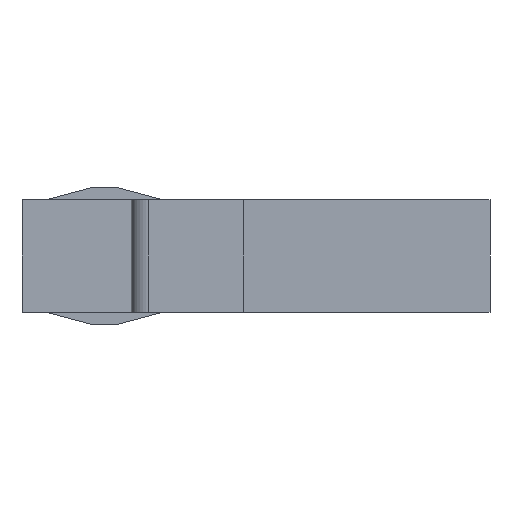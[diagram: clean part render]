
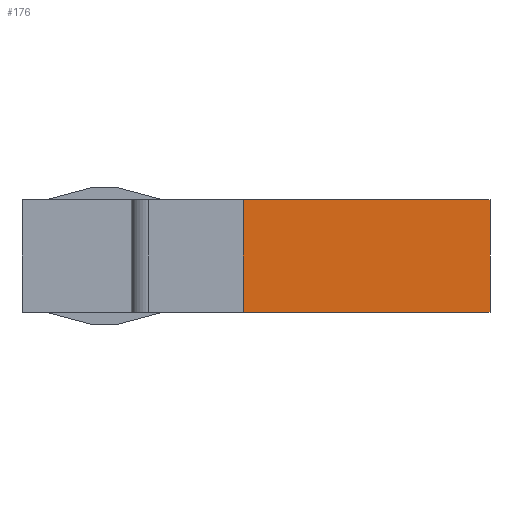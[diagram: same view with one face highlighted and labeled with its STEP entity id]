
A CAD part, left-side view. The second image highlights one B-rep face of the part: STEP entity #176.
In plain terms, the highlighted planar face has unit normal (-1, 0, 0).
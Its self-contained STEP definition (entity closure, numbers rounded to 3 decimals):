
#112 = FACE_OUTER_BOUND ( 'NONE', #405, .T. ) ;
#115 = ORIENTED_EDGE ( 'NONE', *, *, #142, .T. ) ;
#142 = EDGE_CURVE ( 'NONE', #905, #1767, #2941, .T. ) ;
#176 = ADVANCED_FACE ( 'NONE', ( #112 ), #1704, .T. ) ;
#278 = CARTESIAN_POINT ( 'NONE',  ( -2.235, 0., 2.54 ) ) ;
#292 = VERTEX_POINT ( 'NONE', #2405 ) ;
#405 = EDGE_LOOP ( 'NONE', ( #3546, #115, #2902, #2027 ) ) ;
#423 = LINE ( 'NONE', #2264, #2037 ) ;
#438 = DIRECTION ( 'NONE',  ( 0., 0., 1. ) ) ;
#489 = DIRECTION ( 'NONE',  ( 0., 1., 0. ) ) ;
#500 = EDGE_CURVE ( 'NONE', #292, #905, #1309, .T. ) ;
#874 = DIRECTION ( 'NONE',  ( 0., 1., 0. ) ) ;
#905 = VERTEX_POINT ( 'NONE', #278 ) ;
#947 = VECTOR ( 'NONE', #3270, 1000. ) ;
#1081 = EDGE_CURVE ( 'NONE', #2437, #292, #423, .T. ) ;
#1309 = LINE ( 'NONE', #2003, #2973 ) ;
#1479 = CARTESIAN_POINT ( 'NONE',  ( -2.235, -11.176, -2.54 ) ) ;
#1633 = CARTESIAN_POINT ( 'NONE',  ( -2.235, 0., 2.54 ) ) ;
#1704 = PLANE ( 'NONE',  #3223 ) ;
#1721 = CARTESIAN_POINT ( 'NONE',  ( -2.235, 0., -2.54 ) ) ;
#1767 = VERTEX_POINT ( 'NONE', #1721 ) ;
#2003 = CARTESIAN_POINT ( 'NONE',  ( -2.235, -11.176, 2.54 ) ) ;
#2027 = ORIENTED_EDGE ( 'NONE', *, *, #1081, .T. ) ;
#2037 = VECTOR ( 'NONE', #2225, 1000. ) ;
#2225 = DIRECTION ( 'NONE',  ( 0., 0., 1. ) ) ;
#2264 = CARTESIAN_POINT ( 'NONE',  ( -2.235, -11.176, -2.54 ) ) ;
#2363 = DIRECTION ( 'NONE',  ( -1., 0., 0. ) ) ;
#2405 = CARTESIAN_POINT ( 'NONE',  ( -2.235, -11.176, 2.54 ) ) ;
#2437 = VERTEX_POINT ( 'NONE', #3572 ) ;
#2496 = EDGE_CURVE ( 'NONE', #2437, #1767, #3077, .T. ) ;
#2670 = CARTESIAN_POINT ( 'NONE',  ( -2.235, -11.176, -2.54 ) ) ;
#2747 = VECTOR ( 'NONE', #874, 1000. ) ;
#2902 = ORIENTED_EDGE ( 'NONE', *, *, #2496, .F. ) ;
#2941 = LINE ( 'NONE', #1633, #947 ) ;
#2973 = VECTOR ( 'NONE', #489, 1000. ) ;
#3077 = LINE ( 'NONE', #1479, #2747 ) ;
#3223 = AXIS2_PLACEMENT_3D ( 'NONE', #2670, #2363, #438 ) ;
#3270 = DIRECTION ( 'NONE',  ( 0., 0., -1. ) ) ;
#3546 = ORIENTED_EDGE ( 'NONE', *, *, #500, .T. ) ;
#3572 = CARTESIAN_POINT ( 'NONE',  ( -2.235, -11.176, -2.54 ) ) ;
